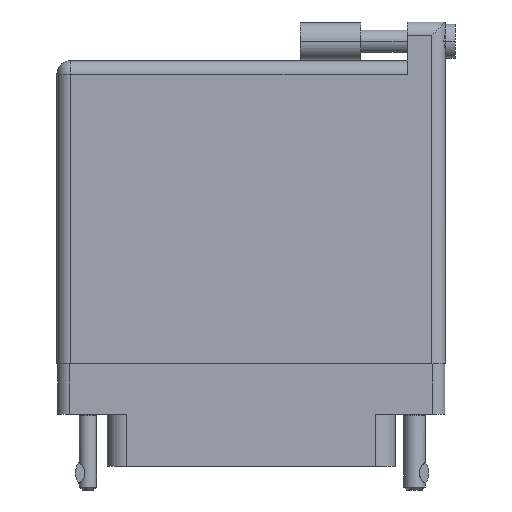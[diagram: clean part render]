
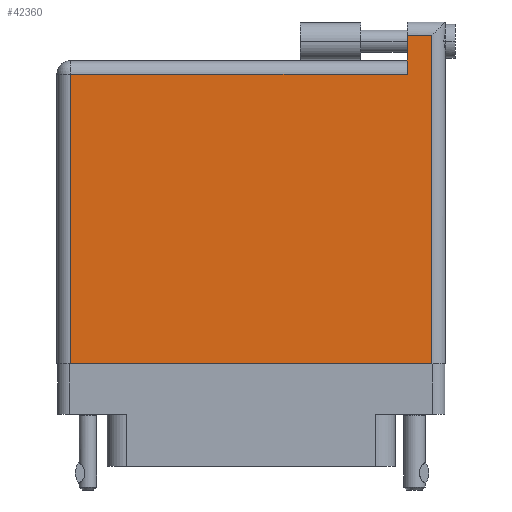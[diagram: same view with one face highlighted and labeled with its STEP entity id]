
A CAD part, front view. The second image highlights one B-rep face of the part: STEP entity #42360.
In plain terms, the highlighted face is planar.
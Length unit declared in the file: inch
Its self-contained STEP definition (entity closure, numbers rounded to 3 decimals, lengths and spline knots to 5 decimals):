
#1264 = VECTOR ( 'NONE', #8835, 39.37008 ) ;
#1734 = CARTESIAN_POINT ( 'NONE',  ( 1.938, 1.696, 0. ) ) ;
#2406 = CARTESIAN_POINT ( 'NONE',  ( 1.938, 1.766, 0. ) ) ;
#3191 = LINE ( 'NONE', #2406, #22313 ) ;
#3385 = CARTESIAN_POINT ( 'NONE',  ( 0., 1.496, 0. ) ) ;
#4263 = VERTEX_POINT ( 'NONE', #15043 ) ;
#4449 = DIRECTION ( 'NONE',  ( 1., 0., 0. ) ) ;
#6038 = EDGE_CURVE ( 'NONE', #4263, #13487, #24503, .T. ) ;
#7409 = VERTEX_POINT ( 'NONE', #18147 ) ;
#7772 = VECTOR ( 'NONE', #13389, 39.37008 ) ;
#8660 = EDGE_CURVE ( 'NONE', #40729, #13156, #30201, .T. ) ;
#8756 = LINE ( 'NONE', #25133, #39983 ) ;
#8835 = DIRECTION ( 'NONE',  ( -1., 0., 0. ) ) ;
#9346 = CARTESIAN_POINT ( 'NONE',  ( 0.07, 0., 0. ) ) ;
#10907 = CARTESIAN_POINT ( 'NONE',  ( 0.07, 0., 0. ) ) ;
#10932 = VECTOR ( 'NONE', #29722, 39.37008 ) ;
#11242 = CARTESIAN_POINT ( 'NONE',  ( 1.811, 1.696, 0. ) ) ;
#13088 = LINE ( 'NONE', #45692, #13679 ) ;
#13156 = VERTEX_POINT ( 'NONE', #11242 ) ;
#13389 = DIRECTION ( 'NONE',  ( 0., -1., 0. ) ) ;
#13487 = VERTEX_POINT ( 'NONE', #10907 ) ;
#13679 = VECTOR ( 'NONE', #4449, 39.37008 ) ;
#15043 = CARTESIAN_POINT ( 'NONE',  ( 0.07, 1.496, 0. ) ) ;
#16147 = AXIS2_PLACEMENT_3D ( 'NONE', #40271, #36863, #32798 ) ;
#16494 = ORIENTED_EDGE ( 'NONE', *, *, #46438, .T. ) ;
#17023 = EDGE_CURVE ( 'NONE', #47677, #40729, #3191, .T. ) ;
#18147 = CARTESIAN_POINT ( 'NONE',  ( 1.811, 1.496, 0. ) ) ;
#20228 = EDGE_CURVE ( 'NONE', #13156, #7409, #8756, .T. ) ;
#20793 = ORIENTED_EDGE ( 'NONE', *, *, #20228, .T. ) ;
#21951 = PLANE ( 'NONE',  #16147 ) ;
#22313 = VECTOR ( 'NONE', #24998, 39.37008 ) ;
#22834 = EDGE_CURVE ( 'NONE', #7409, #4263, #29984, .T. ) ;
#24021 = ORIENTED_EDGE ( 'NONE', *, *, #22834, .T. ) ;
#24503 = LINE ( 'NONE', #9346, #7772 ) ;
#24998 = DIRECTION ( 'NONE',  ( 0., 1., 0. ) ) ;
#25133 = CARTESIAN_POINT ( 'NONE',  ( 1.811, 1.766, 0. ) ) ;
#25644 = ORIENTED_EDGE ( 'NONE', *, *, #8660, .T. ) ;
#28018 = EDGE_LOOP ( 'NONE', ( #16494, #41212, #25644, #20793, #24021, #41709 ) ) ;
#28733 = DIRECTION ( 'NONE',  ( 0., -1., 0. ) ) ;
#29722 = DIRECTION ( 'NONE',  ( -1., 0., 0. ) ) ;
#29984 = LINE ( 'NONE', #3385, #10932 ) ;
#30201 = LINE ( 'NONE', #42590, #1264 ) ;
#32798 = DIRECTION ( 'NONE',  ( -1., 0., 0. ) ) ;
#36863 = DIRECTION ( 'NONE',  ( 0., 0., -1. ) ) ;
#36950 = FACE_OUTER_BOUND ( 'NONE', #28018, .T. ) ;
#39556 = CARTESIAN_POINT ( 'NONE',  ( 1.938, 0., 0. ) ) ;
#39983 = VECTOR ( 'NONE', #28733, 39.37008 ) ;
#40271 = CARTESIAN_POINT ( 'NONE',  ( 0., 1.566, 0. ) ) ;
#40729 = VERTEX_POINT ( 'NONE', #1734 ) ;
#41212 = ORIENTED_EDGE ( 'NONE', *, *, #17023, .T. ) ;
#41709 = ORIENTED_EDGE ( 'NONE', *, *, #6038, .T. ) ;
#42360 = ADVANCED_FACE ( 'NONE', ( #36950 ), #21951, .F. ) ;
#42590 = CARTESIAN_POINT ( 'NONE',  ( 0., 1.696, 0. ) ) ;
#45692 = CARTESIAN_POINT ( 'NONE',  ( 0., 0., 0. ) ) ;
#46438 = EDGE_CURVE ( 'NONE', #13487, #47677, #13088, .T. ) ;
#47677 = VERTEX_POINT ( 'NONE', #39556 ) ;
